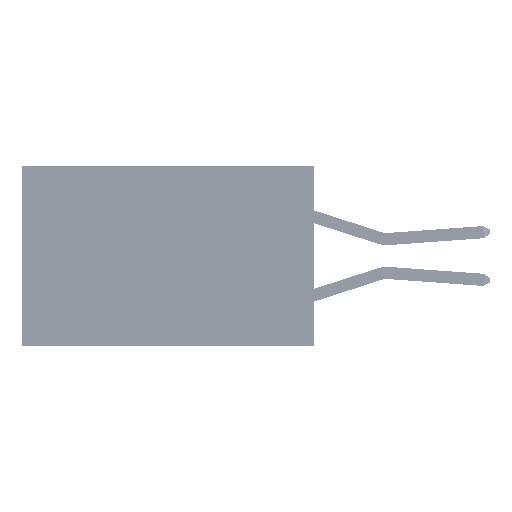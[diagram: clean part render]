
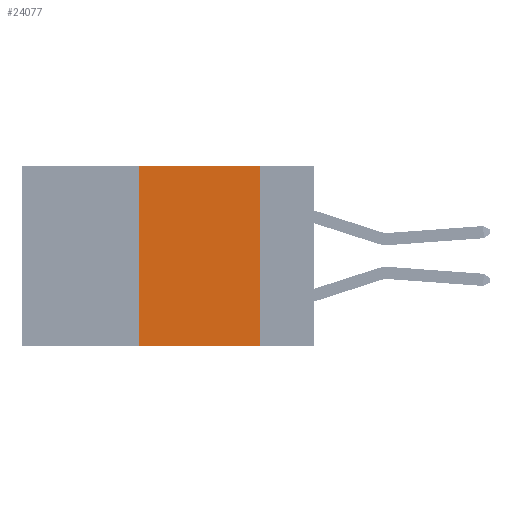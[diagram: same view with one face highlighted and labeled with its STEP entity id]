
A CAD part, left-side view. The second image highlights one B-rep face of the part: STEP entity #24077.
In plain terms, the highlighted planar face has unit normal (-1, 0, 0).
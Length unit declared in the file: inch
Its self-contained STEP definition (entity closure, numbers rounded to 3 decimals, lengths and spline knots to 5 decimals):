
#380 = EDGE_LOOP ( 'NONE', ( #31307, #29823, #3648, #27446 ) ) ;
#1425 = CARTESIAN_POINT ( 'NONE',  ( 0., 0.36, -0.37 ) ) ;
#1924 = DIRECTION ( 'NONE',  ( 0., -1., 0. ) ) ;
#3010 = CARTESIAN_POINT ( 'NONE',  ( 0., 0.11, 0. ) ) ;
#3520 = VECTOR ( 'NONE', #1924, 39.37008 ) ;
#3648 = ORIENTED_EDGE ( 'NONE', *, *, #41881, .F. ) ;
#5971 = EDGE_CURVE ( 'NONE', #27983, #17678, #13982, .T. ) ;
#7913 = CARTESIAN_POINT ( 'NONE',  ( 0., 0.11, 0. ) ) ;
#8429 = LINE ( 'NONE', #36768, #34628 ) ;
#13464 = CARTESIAN_POINT ( 'NONE',  ( 0., 0.6, -0.37 ) ) ;
#13982 = LINE ( 'NONE', #13464, #3520 ) ;
#14111 = AXIS2_PLACEMENT_3D ( 'NONE', #40983, #40813, #22797 ) ;
#14253 = DIRECTION ( 'NONE',  ( 0., 0., -1. ) ) ;
#17678 = VERTEX_POINT ( 'NONE', #27149 ) ;
#19054 = PLANE ( 'NONE',  #14111 ) ;
#19597 = LINE ( 'NONE', #3010, #41658 ) ;
#22797 = DIRECTION ( 'NONE',  ( 0., 0., -1. ) ) ;
#23414 = DIRECTION ( 'NONE',  ( 0., -1., 0. ) ) ;
#23976 = FACE_OUTER_BOUND ( 'NONE', #380, .T. ) ;
#24077 = ADVANCED_FACE ( 'NONE', ( #23976 ), #19054, .F. ) ;
#27149 = CARTESIAN_POINT ( 'NONE',  ( 0., 0.11, -0.37 ) ) ;
#27446 = ORIENTED_EDGE ( 'NONE', *, *, #5971, .T. ) ;
#27983 = VERTEX_POINT ( 'NONE', #1425 ) ;
#29121 = VECTOR ( 'NONE', #23414, 39.37008 ) ;
#29254 = EDGE_CURVE ( 'NONE', #30470, #40848, #35522, .T. ) ;
#29823 = ORIENTED_EDGE ( 'NONE', *, *, #29254, .F. ) ;
#30273 = CARTESIAN_POINT ( 'NONE',  ( 0., 0.6, 0. ) ) ;
#30470 = VERTEX_POINT ( 'NONE', #36679 ) ;
#31307 = ORIENTED_EDGE ( 'NONE', *, *, #34449, .F. ) ;
#34449 = EDGE_CURVE ( 'NONE', #40848, #17678, #19597, .T. ) ;
#34628 = VECTOR ( 'NONE', #36601, 39.37008 ) ;
#35522 = LINE ( 'NONE', #30273, #29121 ) ;
#36601 = DIRECTION ( 'NONE',  ( 0., 0., 1. ) ) ;
#36679 = CARTESIAN_POINT ( 'NONE',  ( 0., 0.36, 0. ) ) ;
#36768 = CARTESIAN_POINT ( 'NONE',  ( 0., 0.36, 0. ) ) ;
#40813 = DIRECTION ( 'NONE',  ( 1., 0., 0. ) ) ;
#40848 = VERTEX_POINT ( 'NONE', #7913 ) ;
#40983 = CARTESIAN_POINT ( 'NONE',  ( 0., 0.6, 0. ) ) ;
#41658 = VECTOR ( 'NONE', #14253, 39.37008 ) ;
#41881 = EDGE_CURVE ( 'NONE', #27983, #30470, #8429, .T. ) ;
